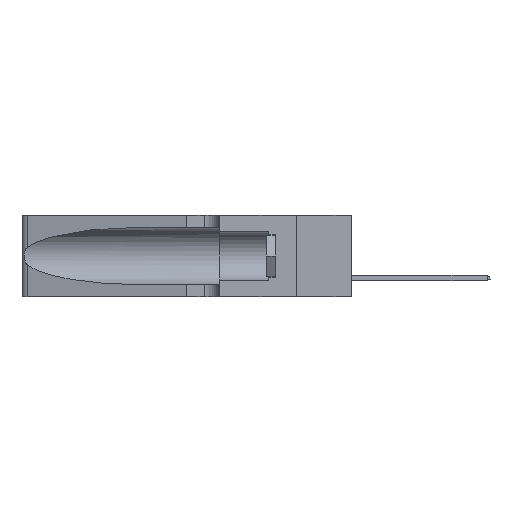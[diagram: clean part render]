
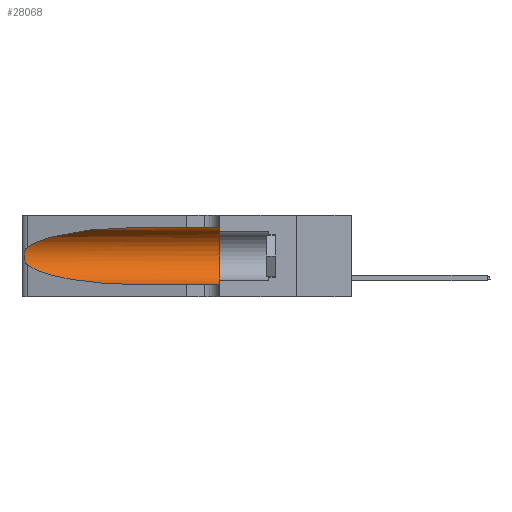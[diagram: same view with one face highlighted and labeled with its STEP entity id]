
A CAD part, left-side view. The second image highlights one B-rep face of the part: STEP entity #28068.
In plain terms, the highlighted cylindrical face has radius 3.308 mm (diameter 6.617 mm), a partial arc.
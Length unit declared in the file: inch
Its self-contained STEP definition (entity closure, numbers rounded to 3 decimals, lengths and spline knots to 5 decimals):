
#282 = ORIENTED_EDGE ( 'NONE', *, *, #16163, .T. ) ;
#592 = CIRCLE ( 'NONE', #8853, 0.13025 ) ;
#891 = CARTESIAN_POINT ( 'NONE',  ( 0.1305, 1.61858, 0.05475 ) ) ;
#2052 = CARTESIAN_POINT ( 'NONE',  ( 0.25789, 1.23486, 0.15765 ) ) ;
#2355 = CARTESIAN_POINT ( 'NONE',  ( 0.25639, 1.23184, 0.21858 ) ) ;
#2462 = CARTESIAN_POINT ( 'NONE',  ( 0.1305, 0.35, 0.185 ) ) ;
#3543 = EDGE_CURVE ( 'NONE', #5517, #10753, #5633, .T. ) ;
#3611 = CARTESIAN_POINT ( 'NONE',  ( 0.2373, 1.15595, 0.08982 ) ) ;
#3654 = VECTOR ( 'NONE', #7979, 39.37008 ) ;
#3812 = CARTESIAN_POINT ( 'NONE',  ( 0.1305, 0.72297, 0.05475 ) ) ;
#4309 = CARTESIAN_POINT ( 'NONE',  ( 0.18966, 0.96281, 0.31525 ) ) ;
#4741 = CARTESIAN_POINT ( 'NONE',  ( 0.25487, 1.22718, 0.14631 ) ) ;
#4815 = CARTESIAN_POINT ( 'NONE',  ( 0.2373, 1.15595, 0.28018 ) ) ;
#5517 = VERTEX_POINT ( 'NONE', #18992 ) ;
#5633 = B_SPLINE_CURVE_WITH_KNOTS ( 'NONE', 3,
 ( #9176, #6998, #2355, #18811, #30527, #25740, #11745, #13838, #30421, #16248, #2052, #20888, #21196, #4741 ),
 .UNSPECIFIED., .F., .F.,
 ( 4, 2, 2, 2, 2, 2, 4 ),
 ( 0., 0.00027, 0.00053, 0.00107, 0.0016, 0.00187, 0.00214 ),
 .UNSPECIFIED. ) ;
#6998 = CARTESIAN_POINT ( 'NONE',  ( 0.25555, 1.22994, 0.2215 ) ) ;
#7326 = LINE ( 'NONE', #10338, #3654 ) ;
#7979 = DIRECTION ( 'NONE',  ( 0., -1., 0. ) ) ;
#8126 = AXIS2_PLACEMENT_3D ( 'NONE', #13577, #13484, #18161 ) ;
#8250 = CARTESIAN_POINT ( 'NONE',  ( 0.25487, 1.22718, 0.14631 ) ) ;
#8350 = CARTESIAN_POINT ( 'NONE',  ( 0.18966, 0.96281, 0.05475 ) ) ;
#8802 = EDGE_LOOP ( 'NONE', ( #282, #16211, #9435, #12953, #12140, #17914 ) ) ;
#8853 = AXIS2_PLACEMENT_3D ( 'NONE', #2462, #28357, #19031 ) ;
#9176 = CARTESIAN_POINT ( 'NONE',  ( 0.25487, 1.22718, 0.22369 ) ) ;
#9435 = ORIENTED_EDGE ( 'NONE', *, *, #26643, .T. ) ;
#9711 = EDGE_CURVE ( 'NONE', #27119, #16957, #11074, .T. ) ;
#10262 = EDGE_CURVE ( 'NONE', #16761, #30654, #7326, .T. ) ;
#10338 = CARTESIAN_POINT ( 'NONE',  ( 0.1305, 1.61858, 0.31525 ) ) ;
#10753 = VERTEX_POINT ( 'NONE', #26472 ) ;
#11074 = LINE ( 'NONE', #891, #23309 ) ;
#11745 = CARTESIAN_POINT ( 'NONE',  ( 0.26075, 1.23896, 0.19203 ) ) ;
#12140 = ORIENTED_EDGE ( 'NONE', *, *, #23875, .F. ) ;
#12953 = ORIENTED_EDGE ( 'NONE', *, *, #9711, .T. ) ;
#13182 = CARTESIAN_POINT ( 'NONE',  ( 0.1305, 0.72297, 0.31525 ) ) ;
#13484 = DIRECTION ( 'NONE',  ( 0., -1., 0. ) ) ;
#13577 = CARTESIAN_POINT ( 'NONE',  ( 0.1305, 1.61858, 0.185 ) ) ;
#13838 = CARTESIAN_POINT ( 'NONE',  ( 0.26075, 1.23896, 0.178 ) ) ;
#16163 = EDGE_CURVE ( 'NONE', #16761, #5517, #26293, .T. ) ;
#16211 = ORIENTED_EDGE ( 'NONE', *, *, #3543, .T. ) ;
#16248 = CARTESIAN_POINT ( 'NONE',  ( 0.25856, 1.23593, 0.16098 ) ) ;
#16761 = VERTEX_POINT ( 'NONE', #13182 ) ;
#16957 = VERTEX_POINT ( 'NONE', #27885 ) ;
#17914 = ORIENTED_EDGE ( 'NONE', *, *, #10262, .F. ) ;
#18161 = DIRECTION ( 'NONE',  ( 0., 0., -1. ) ) ;
#18473 = CARTESIAN_POINT ( 'NONE',  ( 0.1305, 0.72297, 0.31525 ) ) ;
#18811 = CARTESIAN_POINT ( 'NONE',  ( 0.25787, 1.23484, 0.2124 ) ) ;
#18872 = CYLINDRICAL_SURFACE ( 'NONE', #8126, 0.13025 ) ;
#18992 = CARTESIAN_POINT ( 'NONE',  ( 0.25487, 1.22718, 0.22369 ) ) ;
#19031 = DIRECTION ( 'NONE',  ( 0., 0., 1. ) ) ;
#20888 = CARTESIAN_POINT ( 'NONE',  ( 0.25639, 1.23186, 0.15144 ) ) ;
#21196 = CARTESIAN_POINT ( 'NONE',  ( 0.25555, 1.22993, 0.14849 ) ) ;
#23309 = VECTOR ( 'NONE', #29474, 39.37008 ) ;
#23626 = CARTESIAN_POINT ( 'NONE',  ( 0.25487, 1.22718, 0.22369 ) ) ;
#23875 = EDGE_CURVE ( 'NONE', #30654, #16957, #592, .T. ) ;
#24908 = CARTESIAN_POINT ( 'NONE',  ( 0.1305, 0.72297, 0.05475 ) ) ;
#25159 = FACE_OUTER_BOUND ( 'NONE', #8802, .T. ) ;
#25740 = CARTESIAN_POINT ( 'NONE',  ( 0.26018, 1.23835, 0.19895 ) ) ;
#26293 =( BOUNDED_CURVE ( )  B_SPLINE_CURVE ( 3, ( #18473, #4309, #4815, #23626 ),
 .UNSPECIFIED., .F., .T. ) 
 B_SPLINE_CURVE_WITH_KNOTS ( ( 4, 4 ),
 ( 1.5708, 2.84003 ),
 .UNSPECIFIED. ) 
 CURVE ( )  GEOMETRIC_REPRESENTATION_ITEM ( )  RATIONAL_B_SPLINE_CURVE ( ( 1., 0.87, 0.87, 1. ) ) 
 REPRESENTATION_ITEM ( '' )  );
#26472 = CARTESIAN_POINT ( 'NONE',  ( 0.25487, 1.22718, 0.14631 ) ) ;
#26643 = EDGE_CURVE ( 'NONE', #10753, #27119, #26676, .T. ) ;
#26676 =( BOUNDED_CURVE ( )  B_SPLINE_CURVE ( 3, ( #8250, #3611, #8350, #24908 ),
 .UNSPECIFIED., .F., .F. ) 
 B_SPLINE_CURVE_WITH_KNOTS ( ( 4, 4 ),
 ( 3.44316, 4.71239 ),
 .UNSPECIFIED. ) 
 CURVE ( )  GEOMETRIC_REPRESENTATION_ITEM ( )  RATIONAL_B_SPLINE_CURVE ( ( 1., 0.87, 0.87, 1. ) ) 
 REPRESENTATION_ITEM ( '' )  );
#27119 = VERTEX_POINT ( 'NONE', #3812 ) ;
#27885 = CARTESIAN_POINT ( 'NONE',  ( 0.1305, 0.35, 0.05475 ) ) ;
#28068 = ADVANCED_FACE ( 'NONE', ( #25159 ), #18872, .F. ) ;
#28357 = DIRECTION ( 'NONE',  ( 0., 1., 0. ) ) ;
#29474 = DIRECTION ( 'NONE',  ( 0., -1., 0. ) ) ;
#29895 = CARTESIAN_POINT ( 'NONE',  ( 0.1305, 0.35, 0.31525 ) ) ;
#30421 = CARTESIAN_POINT ( 'NONE',  ( 0.26017, 1.23833, 0.17102 ) ) ;
#30527 = CARTESIAN_POINT ( 'NONE',  ( 0.25854, 1.2359, 0.20912 ) ) ;
#30654 = VERTEX_POINT ( 'NONE', #29895 ) ;
